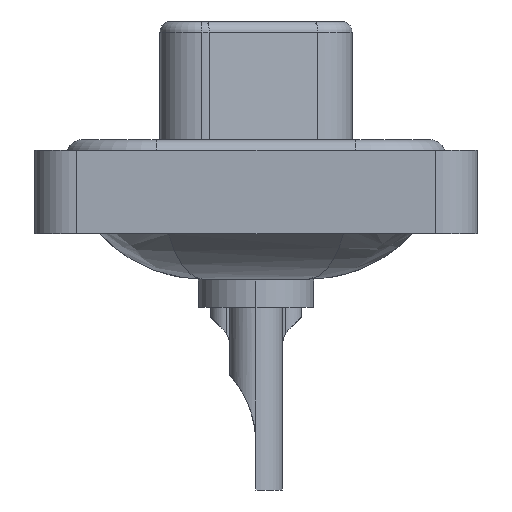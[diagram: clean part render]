
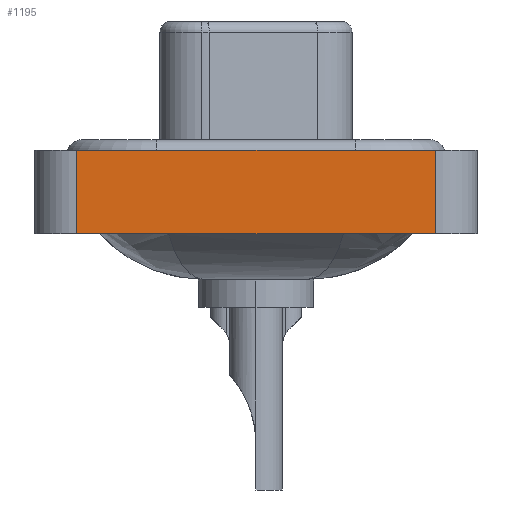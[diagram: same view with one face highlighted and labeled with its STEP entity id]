
A CAD part, left-side view. The second image highlights one B-rep face of the part: STEP entity #1195.
In plain terms, the highlighted planar face has unit normal (-1, 0, 0).
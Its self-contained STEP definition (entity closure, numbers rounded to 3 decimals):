
#1108 = ORIENTED_EDGE ( 'NONE', *, *, #4958, .F. ) ;
#1195 = ADVANCED_FACE ( 'NONE', ( #21554 ), #18371, .T. ) ;
#2601 = VECTOR ( 'NONE', #18332, 1000. ) ;
#3433 = EDGE_CURVE ( 'NONE', #3765, #11979, #15272, .T. ) ;
#3724 = CARTESIAN_POINT ( 'NONE',  ( -7.35, -8.55, 0.4 ) ) ;
#3732 = EDGE_CURVE ( 'NONE', #16051, #3765, #9256, .T. ) ;
#3765 = VERTEX_POINT ( 'NONE', #7556 ) ;
#4401 = ORIENTED_EDGE ( 'NONE', *, *, #18028, .F. ) ;
#4535 = CARTESIAN_POINT ( 'NONE',  ( -7.35, -8.55, -3.6 ) ) ;
#4958 = EDGE_CURVE ( 'NONE', #18510, #11979, #13802, .T. ) ;
#5220 = VECTOR ( 'NONE', #11372, 1000. ) ;
#6859 = ORIENTED_EDGE ( 'NONE', *, *, #3732, .T. ) ;
#7556 = CARTESIAN_POINT ( 'NONE',  ( -7.35, -8.55, -3.6 ) ) ;
#8812 = CARTESIAN_POINT ( 'NONE',  ( -7.35, -8.55, 0.4 ) ) ;
#9256 = LINE ( 'NONE', #17656, #16740 ) ;
#9469 = CARTESIAN_POINT ( 'NONE',  ( -7.35, 8.55, -3.6 ) ) ;
#9776 = DIRECTION ( 'NONE',  ( -1., 0., 0. ) ) ;
#9777 = LINE ( 'NONE', #16691, #5220 ) ;
#11372 = DIRECTION ( 'NONE',  ( 0., 0., 1. ) ) ;
#11979 = VERTEX_POINT ( 'NONE', #8812 ) ;
#13802 = LINE ( 'NONE', #3724, #15324 ) ;
#13816 = AXIS2_PLACEMENT_3D ( 'NONE', #4535, #9776, #15089 ) ;
#14256 = DIRECTION ( 'NONE',  ( 0., -1., 0. ) ) ;
#14771 = DIRECTION ( 'NONE',  ( 0., -1., 0. ) ) ;
#15089 = DIRECTION ( 'NONE',  ( 0., 0., 1. ) ) ;
#15159 = CARTESIAN_POINT ( 'NONE',  ( -7.35, -8.55, -3.6 ) ) ;
#15272 = LINE ( 'NONE', #15159, #2601 ) ;
#15324 = VECTOR ( 'NONE', #14771, 1000. ) ;
#16051 = VERTEX_POINT ( 'NONE', #9469 ) ;
#16691 = CARTESIAN_POINT ( 'NONE',  ( -7.35, 8.55, -3.6 ) ) ;
#16740 = VECTOR ( 'NONE', #14256, 1000. ) ;
#17656 = CARTESIAN_POINT ( 'NONE',  ( -7.35, -8.55, -3.6 ) ) ;
#18028 = EDGE_CURVE ( 'NONE', #16051, #18510, #9777, .T. ) ;
#18332 = DIRECTION ( 'NONE',  ( 0., 0., 1. ) ) ;
#18371 = PLANE ( 'NONE',  #13816 ) ;
#18510 = VERTEX_POINT ( 'NONE', #22334 ) ;
#21554 = FACE_OUTER_BOUND ( 'NONE', #22298, .T. ) ;
#21973 = ORIENTED_EDGE ( 'NONE', *, *, #3433, .T. ) ;
#22298 = EDGE_LOOP ( 'NONE', ( #21973, #1108, #4401, #6859 ) ) ;
#22334 = CARTESIAN_POINT ( 'NONE',  ( -7.35, 8.55, 0.4 ) ) ;
